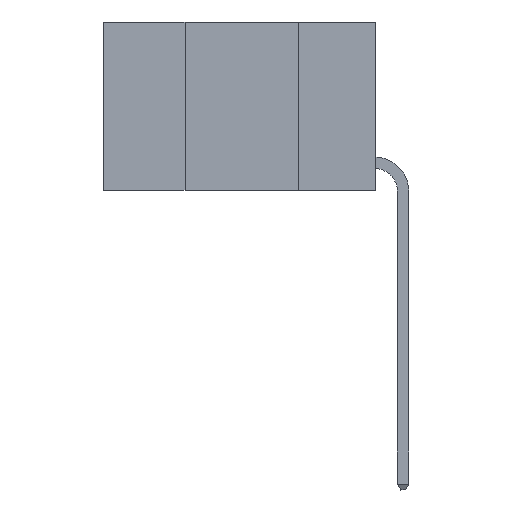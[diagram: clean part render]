
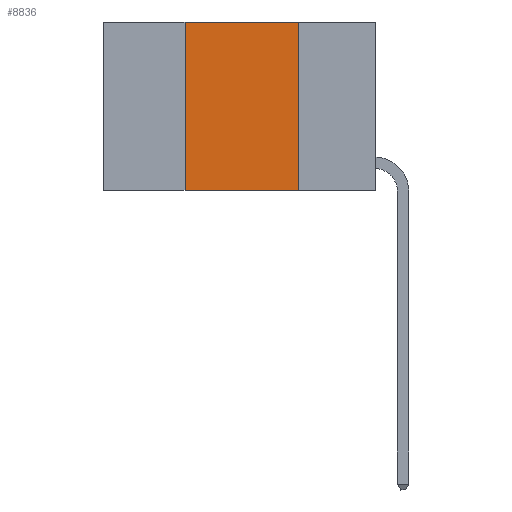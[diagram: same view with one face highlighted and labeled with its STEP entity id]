
A CAD part, left-side view. The second image highlights one B-rep face of the part: STEP entity #8836.
In plain terms, the highlighted planar face has unit normal (-1, 0, 0).
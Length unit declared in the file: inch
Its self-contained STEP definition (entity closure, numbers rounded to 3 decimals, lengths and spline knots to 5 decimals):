
#248 = VECTOR ( 'NONE', #5378, 39.37008 ) ;
#2208 = DIRECTION ( 'NONE',  ( 0., -1., 0. ) ) ;
#2351 = LINE ( 'NONE', #20730, #13148 ) ;
#3162 = VERTEX_POINT ( 'NONE', #21421 ) ;
#3261 = AXIS2_PLACEMENT_3D ( 'NONE', #6029, #22424, #24453 ) ;
#3500 = LINE ( 'NONE', #26353, #248 ) ;
#4166 = EDGE_LOOP ( 'NONE', ( #15668, #15369, #22449, #16667 ) ) ;
#4557 = CARTESIAN_POINT ( 'NONE',  ( 0., 0.17, 0. ) ) ;
#4625 = VERTEX_POINT ( 'NONE', #17516 ) ;
#5322 = CARTESIAN_POINT ( 'NONE',  ( 0., 0.17, 0. ) ) ;
#5378 = DIRECTION ( 'NONE',  ( 0., -1., 0. ) ) ;
#5602 = EDGE_CURVE ( 'NONE', #25055, #4625, #6832, .T. ) ;
#6029 = CARTESIAN_POINT ( 'NONE',  ( 0., 0.6, 0. ) ) ;
#6832 = LINE ( 'NONE', #25666, #13385 ) ;
#8836 = ADVANCED_FACE ( 'NONE', ( #22150 ), #24309, .F. ) ;
#11173 = CARTESIAN_POINT ( 'NONE',  ( 0., 0.42, -0.37 ) ) ;
#13078 = DIRECTION ( 'NONE',  ( 0., 0., 1. ) ) ;
#13148 = VECTOR ( 'NONE', #2208, 39.37008 ) ;
#13385 = VECTOR ( 'NONE', #13078, 39.37008 ) ;
#15369 = ORIENTED_EDGE ( 'NONE', *, *, #19489, .F. ) ;
#15668 = ORIENTED_EDGE ( 'NONE', *, *, #22392, .F. ) ;
#16667 = ORIENTED_EDGE ( 'NONE', *, *, #18881, .T. ) ;
#17516 = CARTESIAN_POINT ( 'NONE',  ( 0., 0.42, 0. ) ) ;
#17639 = DIRECTION ( 'NONE',  ( 0., 0., -1. ) ) ;
#18469 = VECTOR ( 'NONE', #17639, 39.37008 ) ;
#18881 = EDGE_CURVE ( 'NONE', #25055, #3162, #2351, .T. ) ;
#19489 = EDGE_CURVE ( 'NONE', #4625, #21020, #3500, .T. ) ;
#20730 = CARTESIAN_POINT ( 'NONE',  ( 0., 0.6, -0.37 ) ) ;
#21020 = VERTEX_POINT ( 'NONE', #4557 ) ;
#21421 = CARTESIAN_POINT ( 'NONE',  ( 0., 0.17, -0.37 ) ) ;
#22150 = FACE_OUTER_BOUND ( 'NONE', #4166, .T. ) ;
#22392 = EDGE_CURVE ( 'NONE', #21020, #3162, #25752, .T. ) ;
#22424 = DIRECTION ( 'NONE',  ( 1., 0., 0. ) ) ;
#22449 = ORIENTED_EDGE ( 'NONE', *, *, #5602, .F. ) ;
#24309 = PLANE ( 'NONE',  #3261 ) ;
#24453 = DIRECTION ( 'NONE',  ( 0., 0., -1. ) ) ;
#25055 = VERTEX_POINT ( 'NONE', #11173 ) ;
#25666 = CARTESIAN_POINT ( 'NONE',  ( 0., 0.42, 0. ) ) ;
#25752 = LINE ( 'NONE', #5322, #18469 ) ;
#26353 = CARTESIAN_POINT ( 'NONE',  ( 0., 0.6, 0. ) ) ;
